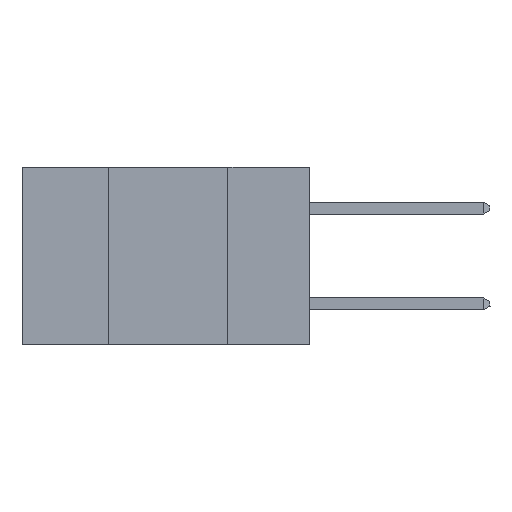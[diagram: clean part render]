
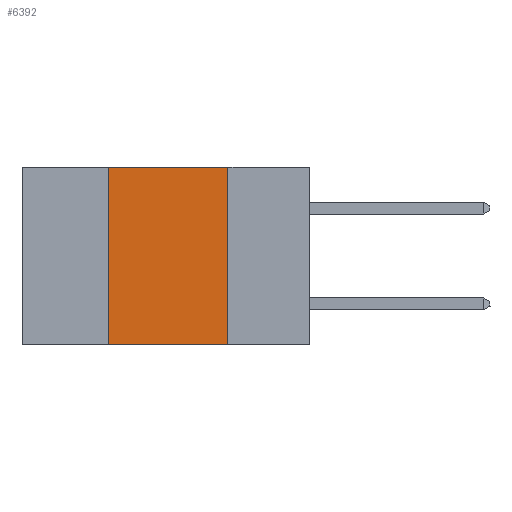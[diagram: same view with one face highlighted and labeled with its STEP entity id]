
A CAD part, left-side view. The second image highlights one B-rep face of the part: STEP entity #6392.
In plain terms, the highlighted planar face has unit normal (-1, 0, 0).
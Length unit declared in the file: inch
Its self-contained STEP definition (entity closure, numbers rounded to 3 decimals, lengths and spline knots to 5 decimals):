
#2162 = DIRECTION ( 'NONE',  ( 0., 0., -1. ) ) ;
#2192 = ORIENTED_EDGE ( 'NONE', *, *, #6687, .F. ) ;
#2891 = VECTOR ( 'NONE', #2162, 39.37008 ) ;
#4969 = VECTOR ( 'NONE', #32616, 39.37008 ) ;
#5245 = VERTEX_POINT ( 'NONE', #6603 ) ;
#6392 = ADVANCED_FACE ( 'NONE', ( #27747 ), #21650, .F. ) ;
#6603 = CARTESIAN_POINT ( 'NONE',  ( 0., 0.42, -0.37 ) ) ;
#6687 = EDGE_CURVE ( 'NONE', #5245, #33622, #17965, .T. ) ;
#7265 = EDGE_CURVE ( 'NONE', #22175, #29829, #9857, .T. ) ;
#8071 = CARTESIAN_POINT ( 'NONE',  ( 0., 0.6, 0. ) ) ;
#8914 = VECTOR ( 'NONE', #26739, 39.37008 ) ;
#9857 = LINE ( 'NONE', #27088, #2891 ) ;
#10925 = AXIS2_PLACEMENT_3D ( 'NONE', #21414, #21882, #24318 ) ;
#13346 = ORIENTED_EDGE ( 'NONE', *, *, #27812, .T. ) ;
#14482 = CARTESIAN_POINT ( 'NONE',  ( 0., 0.42, 0. ) ) ;
#15201 = CARTESIAN_POINT ( 'NONE',  ( 0., 0.42, 0. ) ) ;
#16021 = EDGE_LOOP ( 'NONE', ( #27197, #24012, #2192, #13346 ) ) ;
#16245 = CARTESIAN_POINT ( 'NONE',  ( 0., 0.6, -0.37 ) ) ;
#17965 = LINE ( 'NONE', #14482, #4969 ) ;
#18013 = LINE ( 'NONE', #8071, #28965 ) ;
#18179 = DIRECTION ( 'NONE',  ( 0., -1., 0. ) ) ;
#21414 = CARTESIAN_POINT ( 'NONE',  ( 0., 0.6, 0. ) ) ;
#21650 = PLANE ( 'NONE',  #10925 ) ;
#21882 = DIRECTION ( 'NONE',  ( 1., 0., 0. ) ) ;
#22175 = VERTEX_POINT ( 'NONE', #31098 ) ;
#23067 = CARTESIAN_POINT ( 'NONE',  ( 0., 0.17, -0.37 ) ) ;
#24012 = ORIENTED_EDGE ( 'NONE', *, *, #31070, .F. ) ;
#24318 = DIRECTION ( 'NONE',  ( 0., 0., -1. ) ) ;
#26739 = DIRECTION ( 'NONE',  ( 0., -1., 0. ) ) ;
#27088 = CARTESIAN_POINT ( 'NONE',  ( 0., 0.17, 0. ) ) ;
#27197 = ORIENTED_EDGE ( 'NONE', *, *, #7265, .F. ) ;
#27747 = FACE_OUTER_BOUND ( 'NONE', #16021, .T. ) ;
#27812 = EDGE_CURVE ( 'NONE', #5245, #29829, #31227, .T. ) ;
#28965 = VECTOR ( 'NONE', #18179, 39.37008 ) ;
#29829 = VERTEX_POINT ( 'NONE', #23067 ) ;
#31070 = EDGE_CURVE ( 'NONE', #33622, #22175, #18013, .T. ) ;
#31098 = CARTESIAN_POINT ( 'NONE',  ( 0., 0.17, 0. ) ) ;
#31227 = LINE ( 'NONE', #16245, #8914 ) ;
#32616 = DIRECTION ( 'NONE',  ( 0., 0., 1. ) ) ;
#33622 = VERTEX_POINT ( 'NONE', #15201 ) ;
